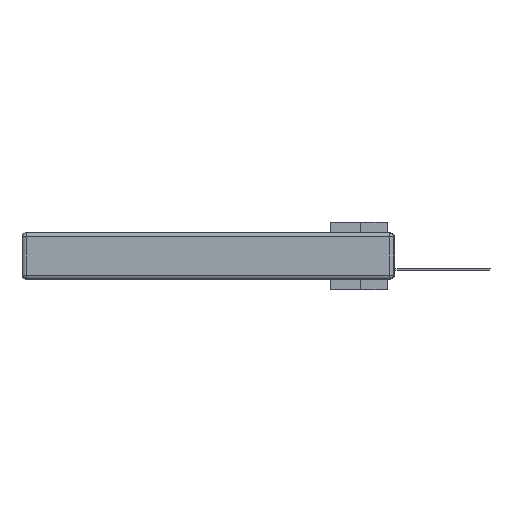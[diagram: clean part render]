
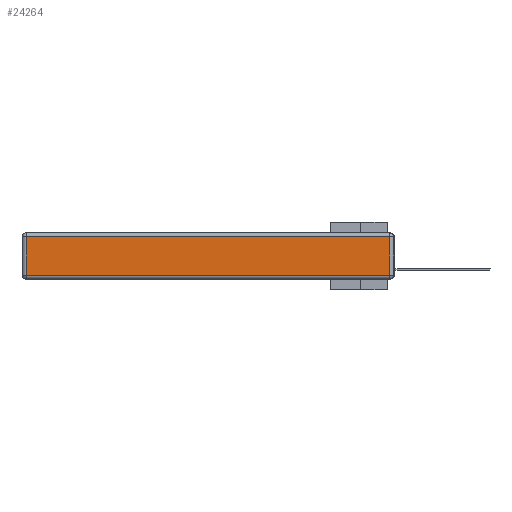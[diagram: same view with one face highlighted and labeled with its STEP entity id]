
A CAD part, left-side view. The second image highlights one B-rep face of the part: STEP entity #24264.
In plain terms, the highlighted planar face has unit normal (-1, 0, 0).
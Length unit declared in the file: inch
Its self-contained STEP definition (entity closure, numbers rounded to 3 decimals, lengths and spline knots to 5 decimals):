
#479 = DIRECTION ( 'NONE',  ( 0., 1., 0. ) ) ;
#1410 = LINE ( 'NONE', #29162, #34874 ) ;
#1601 = DIRECTION ( 'NONE',  ( 0., 0., -1. ) ) ;
#2989 = EDGE_CURVE ( 'NONE', #19816, #19894, #5662, .T. ) ;
#3117 = ORIENTED_EDGE ( 'NONE', *, *, #33301, .T. ) ;
#5492 = LINE ( 'NONE', #16768, #15713 ) ;
#5662 = LINE ( 'NONE', #14524, #12671 ) ;
#5975 = CARTESIAN_POINT ( 'NONE',  ( 0., 2.72, -0.313 ) ) ;
#6685 = ORIENTED_EDGE ( 'NONE', *, *, #19929, .T. ) ;
#7355 = CARTESIAN_POINT ( 'NONE',  ( 0., 0.03, -0.03 ) ) ;
#8013 = ORIENTED_EDGE ( 'NONE', *, *, #2989, .T. ) ;
#12671 = VECTOR ( 'NONE', #479, 39.37008 ) ;
#14200 = VERTEX_POINT ( 'NONE', #5975 ) ;
#14524 = CARTESIAN_POINT ( 'NONE',  ( 0., 2.75, -0.03 ) ) ;
#15713 = VECTOR ( 'NONE', #25480, 39.37008 ) ;
#16343 = ORIENTED_EDGE ( 'NONE', *, *, #26601, .T. ) ;
#16669 = CARTESIAN_POINT ( 'NONE',  ( 0., 0., -0.343 ) ) ;
#16768 = CARTESIAN_POINT ( 'NONE',  ( 0., 0., -0.313 ) ) ;
#19816 = VERTEX_POINT ( 'NONE', #7355 ) ;
#19894 = VERTEX_POINT ( 'NONE', #32884 ) ;
#19929 = EDGE_CURVE ( 'NONE', #35176, #19816, #25489, .T. ) ;
#24264 = ADVANCED_FACE ( 'NONE', ( #34350 ), #29009, .T. ) ;
#25480 = DIRECTION ( 'NONE',  ( 0., -1., 0. ) ) ;
#25489 = LINE ( 'NONE', #33432, #33369 ) ;
#26601 = EDGE_CURVE ( 'NONE', #19894, #14200, #1410, .T. ) ;
#26678 = EDGE_LOOP ( 'NONE', ( #3117, #6685, #8013, #16343 ) ) ;
#27967 = DIRECTION ( 'NONE',  ( 0., 0., 1. ) ) ;
#28264 = DIRECTION ( 'NONE',  ( 0., 0., 1. ) ) ;
#29009 = PLANE ( 'NONE',  #31299 ) ;
#29041 = CARTESIAN_POINT ( 'NONE',  ( 0., 0.03, -0.313 ) ) ;
#29162 = CARTESIAN_POINT ( 'NONE',  ( 0., 2.72, -0.343 ) ) ;
#31299 = AXIS2_PLACEMENT_3D ( 'NONE', #16669, #31779, #27967 ) ;
#31779 = DIRECTION ( 'NONE',  ( -1., 0., 0. ) ) ;
#32884 = CARTESIAN_POINT ( 'NONE',  ( 0., 2.72, -0.03 ) ) ;
#33301 = EDGE_CURVE ( 'NONE', #14200, #35176, #5492, .T. ) ;
#33369 = VECTOR ( 'NONE', #28264, 39.37008 ) ;
#33432 = CARTESIAN_POINT ( 'NONE',  ( 0., 0.03, -0.343 ) ) ;
#34350 = FACE_OUTER_BOUND ( 'NONE', #26678, .T. ) ;
#34874 = VECTOR ( 'NONE', #1601, 39.37008 ) ;
#35176 = VERTEX_POINT ( 'NONE', #29041 ) ;
